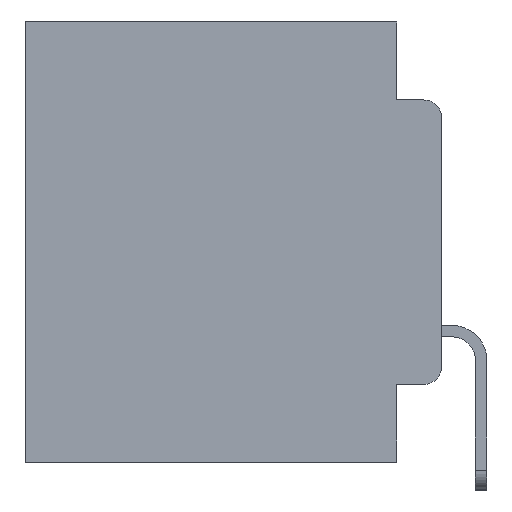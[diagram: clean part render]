
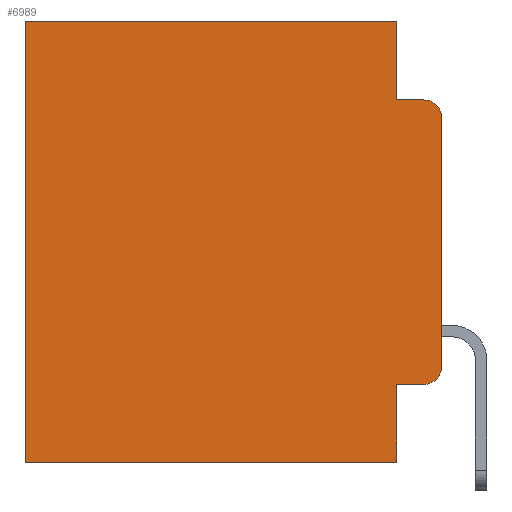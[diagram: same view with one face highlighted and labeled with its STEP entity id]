
A CAD part, left-side view. The second image highlights one B-rep face of the part: STEP entity #6989.
In plain terms, the highlighted planar face has unit normal (-1, 0, 0).
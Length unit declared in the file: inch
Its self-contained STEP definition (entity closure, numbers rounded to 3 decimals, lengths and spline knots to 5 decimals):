
#135 = CARTESIAN_POINT ( 'NONE',  ( 0.298, 0., -0.5 ) ) ;
#348 = DIRECTION ( 'NONE',  ( 0., 0., -1. ) ) ;
#1225 = VECTOR ( 'NONE', #27504, 39.37008 ) ;
#1403 = VECTOR ( 'NONE', #10001, 39.37008 ) ;
#1894 = LINE ( 'NONE', #12459, #1225 ) ;
#1898 = CARTESIAN_POINT ( 'NONE',  ( 0.298, 0.051, -0.5 ) ) ;
#2033 = VECTOR ( 'NONE', #6134, 39.37008 ) ;
#2106 = EDGE_LOOP ( 'NONE', ( #12406, #11713, #23070, #3708, #3088, #23957, #26370, #10720, #18988, #15338 ) ) ;
#2789 = VERTEX_POINT ( 'NONE', #16448 ) ;
#3064 = DIRECTION ( 'NONE',  ( 0., 0., -1. ) ) ;
#3088 = ORIENTED_EDGE ( 'NONE', *, *, #20213, .T. ) ;
#3708 = ORIENTED_EDGE ( 'NONE', *, *, #26148, .F. ) ;
#4563 = EDGE_CURVE ( 'NONE', #18229, #8692, #18428, .T. ) ;
#4717 = DIRECTION ( 'NONE',  ( -1., 0., 0. ) ) ;
#5117 = CARTESIAN_POINT ( 'NONE',  ( 0.298, 0.02, -0.1085 ) ) ;
#6134 = DIRECTION ( 'NONE',  ( 0., 0., -1. ) ) ;
#6511 = CARTESIAN_POINT ( 'NONE',  ( 0.298, 0., -0.1085 ) ) ;
#6534 = FACE_OUTER_BOUND ( 'NONE', #2106, .T. ) ;
#6652 = VECTOR ( 'NONE', #22225, 39.37008 ) ;
#6989 = ADVANCED_FACE ( 'NONE', ( #6534 ), #12393, .F. ) ;
#7130 = CARTESIAN_POINT ( 'NONE',  ( 0.298, 0.473, 0. ) ) ;
#7191 = VERTEX_POINT ( 'NONE', #15734 ) ;
#7364 = DIRECTION ( 'NONE',  ( -1., 0., 0. ) ) ;
#7441 = VECTOR ( 'NONE', #13193, 39.37008 ) ;
#7796 = VERTEX_POINT ( 'NONE', #20097 ) ;
#7923 = CIRCLE ( 'NONE', #9133, 0.02 ) ;
#8293 = CARTESIAN_POINT ( 'NONE',  ( 0.298, 0., 0. ) ) ;
#8564 = DIRECTION ( 'NONE',  ( 0., 0., -1. ) ) ;
#8692 = VERTEX_POINT ( 'NONE', #22275 ) ;
#8845 = CARTESIAN_POINT ( 'NONE',  ( 0.298, 0.02, -0.3915 ) ) ;
#9133 = AXIS2_PLACEMENT_3D ( 'NONE', #5117, #7364, #3064 ) ;
#9162 = DIRECTION ( 'NONE',  ( 0., -1., 0. ) ) ;
#9202 = VECTOR ( 'NONE', #17241, 39.37008 ) ;
#9217 = CARTESIAN_POINT ( 'NONE',  ( 0.298, 0.02, -0.4115 ) ) ;
#9665 = CARTESIAN_POINT ( 'NONE',  ( 0.298, 0.051, -0.4115 ) ) ;
#10001 = DIRECTION ( 'NONE',  ( 0., 1., 0. ) ) ;
#10098 = LINE ( 'NONE', #25601, #22827 ) ;
#10245 = EDGE_CURVE ( 'NONE', #21443, #7796, #10858, .T. ) ;
#10340 = CARTESIAN_POINT ( 'NONE',  ( 0.298, 0., 0. ) ) ;
#10449 = LINE ( 'NONE', #7130, #7441 ) ;
#10720 = ORIENTED_EDGE ( 'NONE', *, *, #19814, .F. ) ;
#10858 = LINE ( 'NONE', #135, #9202 ) ;
#11577 = VECTOR ( 'NONE', #9162, 39.37008 ) ;
#11713 = ORIENTED_EDGE ( 'NONE', *, *, #21900, .T. ) ;
#12393 = PLANE ( 'NONE',  #20791 ) ;
#12406 = ORIENTED_EDGE ( 'NONE', *, *, #4563, .F. ) ;
#12459 = CARTESIAN_POINT ( 'NONE',  ( 0.298, 0.051, -0.0885 ) ) ;
#12520 = DIRECTION ( 'NONE',  ( 0., 0., -1. ) ) ;
#13193 = DIRECTION ( 'NONE',  ( 0., 0., -1. ) ) ;
#13763 = LINE ( 'NONE', #22816, #1403 ) ;
#13989 = CIRCLE ( 'NONE', #19564, 0.02 ) ;
#15338 = ORIENTED_EDGE ( 'NONE', *, *, #15849, .T. ) ;
#15734 = CARTESIAN_POINT ( 'NONE',  ( 0.298, 0.02, -0.0885 ) ) ;
#15849 = EDGE_CURVE ( 'NONE', #24308, #8692, #13989, .T. ) ;
#16448 = CARTESIAN_POINT ( 'NONE',  ( 0.298, 0.051, 0. ) ) ;
#16791 = EDGE_CURVE ( 'NONE', #24115, #7191, #1894, .T. ) ;
#17002 = CARTESIAN_POINT ( 'NONE',  ( 0.298, 0.051, -0.0885 ) ) ;
#17241 = DIRECTION ( 'NONE',  ( 0., 1., 0. ) ) ;
#17278 = LINE ( 'NONE', #19821, #11577 ) ;
#17358 = VERTEX_POINT ( 'NONE', #25312 ) ;
#17650 = EDGE_CURVE ( 'NONE', #21368, #24308, #17278, .T. ) ;
#18229 = VERTEX_POINT ( 'NONE', #6511 ) ;
#18428 = LINE ( 'NONE', #10340, #2033 ) ;
#18988 = ORIENTED_EDGE ( 'NONE', *, *, #17650, .T. ) ;
#19040 = LINE ( 'NONE', #24333, #6652 ) ;
#19375 = EDGE_CURVE ( 'NONE', #17358, #7796, #10449, .T. ) ;
#19564 = AXIS2_PLACEMENT_3D ( 'NONE', #8845, #4717, #348 ) ;
#19814 = EDGE_CURVE ( 'NONE', #21368, #21443, #10098, .T. ) ;
#19821 = CARTESIAN_POINT ( 'NONE',  ( 0.298, 0.051, -0.4115 ) ) ;
#20097 = CARTESIAN_POINT ( 'NONE',  ( 0.298, 0.473, -0.5 ) ) ;
#20213 = EDGE_CURVE ( 'NONE', #2789, #17358, #13763, .T. ) ;
#20791 = AXIS2_PLACEMENT_3D ( 'NONE', #8293, #23259, #8564 ) ;
#21368 = VERTEX_POINT ( 'NONE', #9665 ) ;
#21443 = VERTEX_POINT ( 'NONE', #1898 ) ;
#21900 = EDGE_CURVE ( 'NONE', #18229, #7191, #7923, .T. ) ;
#22225 = DIRECTION ( 'NONE',  ( 0., 0., -1. ) ) ;
#22275 = CARTESIAN_POINT ( 'NONE',  ( 0.298, 0., -0.3915 ) ) ;
#22816 = CARTESIAN_POINT ( 'NONE',  ( 0.298, 0., 0. ) ) ;
#22827 = VECTOR ( 'NONE', #12520, 39.37008 ) ;
#23070 = ORIENTED_EDGE ( 'NONE', *, *, #16791, .F. ) ;
#23259 = DIRECTION ( 'NONE',  ( 1., 0., 0. ) ) ;
#23957 = ORIENTED_EDGE ( 'NONE', *, *, #19375, .T. ) ;
#24115 = VERTEX_POINT ( 'NONE', #17002 ) ;
#24308 = VERTEX_POINT ( 'NONE', #9217 ) ;
#24333 = CARTESIAN_POINT ( 'NONE',  ( 0.298, 0.051, 0. ) ) ;
#25312 = CARTESIAN_POINT ( 'NONE',  ( 0.298, 0.473, 0. ) ) ;
#25601 = CARTESIAN_POINT ( 'NONE',  ( 0.298, 0.051, 0. ) ) ;
#26148 = EDGE_CURVE ( 'NONE', #2789, #24115, #19040, .T. ) ;
#26370 = ORIENTED_EDGE ( 'NONE', *, *, #10245, .F. ) ;
#27504 = DIRECTION ( 'NONE',  ( 0., -1., 0. ) ) ;
